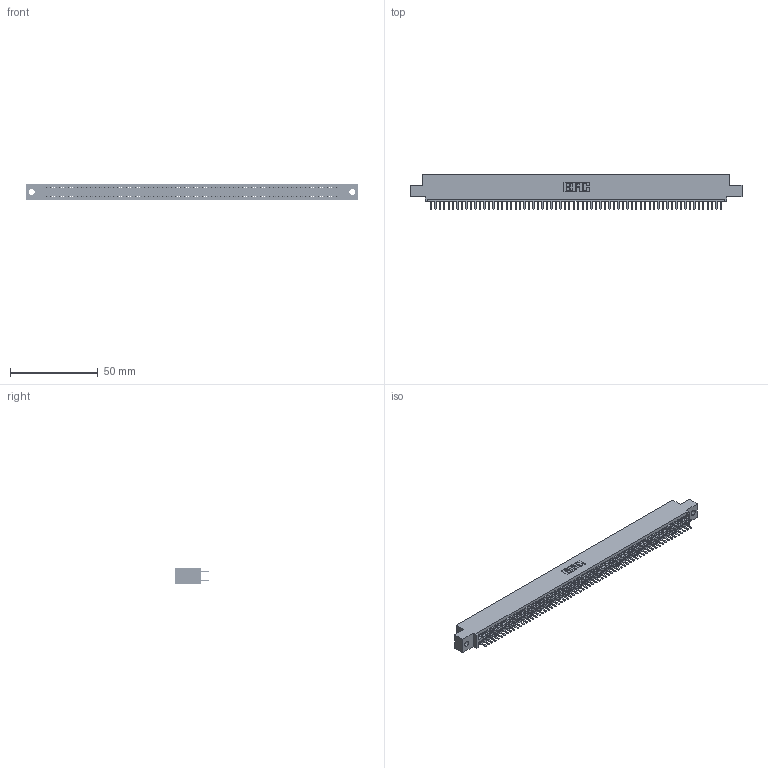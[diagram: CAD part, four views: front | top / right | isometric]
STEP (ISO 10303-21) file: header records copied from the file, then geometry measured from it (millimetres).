
FILE_DESCRIPTION (( 'STEP AP203' ), '1' );
FILE_NAME ('395-132-520-502.STEP', '2018-12-04T20:37:29', ( '' ), ( '' ), 'SwSTEP 2.0', 'SolidWorks 2016', '' );
FILE_SCHEMA (( 'CONFIG_CONTROL_DESIGN' ));
Length unit declared in the file: inch
Products named in the file (3): 345-292-001_345-293-120; 345 Part_0.110 Offset - 0.128 Dia; 395-132-520-502
Assembly tree (133 placements, depth 2):
  395-132-520-502
    345 Part_0.110 Offset - 0.128 Dia
    345-292-001_345-293-120  x132
Bounding box: 188.85 x 19.68 x 9.4 mm (x, y, z)
Volume: 18399.7 mm3; surface area: 27359.3 mm2
Topology: 133 solids, 133 shells, 7258 faces, 21077 edges, 13698 vertices
Faces by surface type: plane 4704, cylinder 2554
Entity records: 48803 total; most frequent: CARTESIAN_POINT 8172, ORIENTED_EDGE 8094, DIRECTION 7163, EDGE_CURVE 4047, LINE 3647, VECTOR 3647, VERTEX_POINT 2694, AXIS2_PLACEMENT_3D 1758
